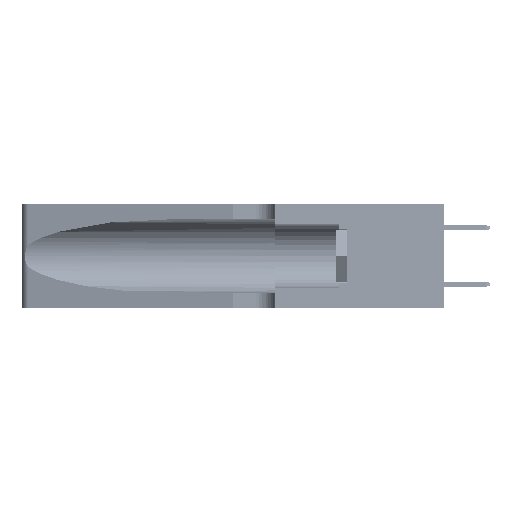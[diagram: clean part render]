
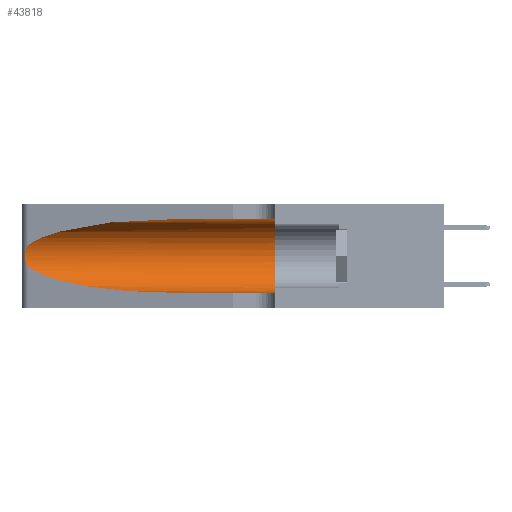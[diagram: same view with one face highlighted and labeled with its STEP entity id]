
A CAD part, left-side view. The second image highlights one B-rep face of the part: STEP entity #43818.
In plain terms, the highlighted cylindrical face has radius 3.308 mm (diameter 6.617 mm), a partial arc.
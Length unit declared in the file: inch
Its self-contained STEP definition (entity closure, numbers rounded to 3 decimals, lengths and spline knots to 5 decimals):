
#5 = AXIS2_PLACEMENT_3D ( 'NONE', #3185, #15823, #49027 ) ;
#410 = LINE ( 'NONE', #9595, #32547 ) ;
#458 = CARTESIAN_POINT ( 'NONE',  ( 0.2373, 1.15595, 0.08982 ) ) ;
#2467 = VERTEX_POINT ( 'NONE', #25370 ) ;
#3185 = CARTESIAN_POINT ( 'NONE',  ( 0.1305, 1.61858, 0.185 ) ) ;
#3196 = DIRECTION ( 'NONE',  ( 0., -1., 0. ) ) ;
#3624 = CARTESIAN_POINT ( 'NONE',  ( 0.25555, 1.22993, 0.14849 ) ) ;
#4055 = AXIS2_PLACEMENT_3D ( 'NONE', #11667, #40899, #15876 ) ;
#4737 = CARTESIAN_POINT ( 'NONE',  ( 0.18966, 0.96281, 0.05475 ) ) ;
#4950 = VERTEX_POINT ( 'NONE', #36254 ) ;
#5387 = B_SPLINE_CURVE_WITH_KNOTS ( 'NONE', 3,
 ( #49276, #53444, #36911, #11862, #41106, #16078, #45245, #20283, #49447, #24527, #53612, #28703, #3624, #32874 ),
 .UNSPECIFIED., .F., .F.,
 ( 4, 2, 2, 2, 2, 2, 4 ),
 ( 0., 0.00027, 0.00053, 0.00107, 0.0016, 0.00187, 0.00214 ),
 .UNSPECIFIED. ) ;
#6263 = CARTESIAN_POINT ( 'NONE',  ( 0.18966, 0.96281, 0.31525 ) ) ;
#9595 = CARTESIAN_POINT ( 'NONE',  ( 0.1305, 1.61858, 0.05475 ) ) ;
#11667 = CARTESIAN_POINT ( 'NONE',  ( 0.1305, 0.35, 0.185 ) ) ;
#11862 = CARTESIAN_POINT ( 'NONE',  ( 0.25787, 1.23484, 0.2124 ) ) ;
#15106 =( BOUNDED_CURVE ( )  B_SPLINE_CURVE ( 3, ( #39679, #6263, #43853, #18870 ),
 .UNSPECIFIED., .F., .F. ) 
 B_SPLINE_CURVE_WITH_KNOTS ( ( 4, 4 ),
 ( 1.5708, 2.84003 ),
 .UNSPECIFIED. ) 
 CURVE ( )  GEOMETRIC_REPRESENTATION_ITEM ( )  RATIONAL_B_SPLINE_CURVE ( ( 1., 0.87, 0.87, 1. ) ) 
 REPRESENTATION_ITEM ( '' )  );
#15823 = DIRECTION ( 'NONE',  ( 0., -1., 0. ) ) ;
#15876 = DIRECTION ( 'NONE',  ( 0., 0., 1. ) ) ;
#16078 = CARTESIAN_POINT ( 'NONE',  ( 0.26018, 1.23835, 0.19895 ) ) ;
#18870 = CARTESIAN_POINT ( 'NONE',  ( 0.25487, 1.22718, 0.22369 ) ) ;
#19521 = VERTEX_POINT ( 'NONE', #27948 ) ;
#20283 = CARTESIAN_POINT ( 'NONE',  ( 0.26075, 1.23896, 0.178 ) ) ;
#21993 = CARTESIAN_POINT ( 'NONE',  ( 0.1305, 0.35, 0.05475 ) ) ;
#24445 = ORIENTED_EDGE ( 'NONE', *, *, #25282, .F. ) ;
#24527 = CARTESIAN_POINT ( 'NONE',  ( 0.25856, 1.23593, 0.16098 ) ) ;
#25282 = EDGE_CURVE ( 'NONE', #19521, #28025, #32556, .T. ) ;
#25370 = CARTESIAN_POINT ( 'NONE',  ( 0.1305, 0.72297, 0.05475 ) ) ;
#26620 = CYLINDRICAL_SURFACE ( 'NONE', #5, 0.13025 ) ;
#26859 = ORIENTED_EDGE ( 'NONE', *, *, #36422, .T. ) ;
#27948 = CARTESIAN_POINT ( 'NONE',  ( 0.1305, 0.35, 0.31525 ) ) ;
#28025 = VERTEX_POINT ( 'NONE', #21993 ) ;
#28703 = CARTESIAN_POINT ( 'NONE',  ( 0.25639, 1.23186, 0.15144 ) ) ;
#29761 = CARTESIAN_POINT ( 'NONE',  ( 0.25487, 1.22718, 0.14631 ) ) ;
#30790 = ORIENTED_EDGE ( 'NONE', *, *, #38462, .T. ) ;
#32547 = VECTOR ( 'NONE', #39021, 39.37008 ) ;
#32556 = CIRCLE ( 'NONE', #4055, 0.13025 ) ;
#32762 = VERTEX_POINT ( 'NONE', #51958 ) ;
#32874 = CARTESIAN_POINT ( 'NONE',  ( 0.25487, 1.22718, 0.14631 ) ) ;
#33967 = CARTESIAN_POINT ( 'NONE',  ( 0.1305, 0.72297, 0.05475 ) ) ;
#33971 = EDGE_CURVE ( 'NONE', #4950, #32762, #15106, .T. ) ;
#35646 = EDGE_LOOP ( 'NONE', ( #36653, #26859, #30790, #45253, #24445, #37536 ) ) ;
#36254 = CARTESIAN_POINT ( 'NONE',  ( 0.1305, 0.72297, 0.31525 ) ) ;
#36422 = EDGE_CURVE ( 'NONE', #32762, #48910, #5387, .T. ) ;
#36653 = ORIENTED_EDGE ( 'NONE', *, *, #33971, .T. ) ;
#36667 = CARTESIAN_POINT ( 'NONE',  ( 0.1305, 1.61858, 0.31525 ) ) ;
#36911 = CARTESIAN_POINT ( 'NONE',  ( 0.25639, 1.23184, 0.21858 ) ) ;
#37184 = LINE ( 'NONE', #36667, #46931 ) ;
#37536 = ORIENTED_EDGE ( 'NONE', *, *, #48543, .F. ) ;
#38462 = EDGE_CURVE ( 'NONE', #48910, #2467, #49846, .T. ) ;
#39021 = DIRECTION ( 'NONE',  ( 0., -1., 0. ) ) ;
#39679 = CARTESIAN_POINT ( 'NONE',  ( 0.1305, 0.72297, 0.31525 ) ) ;
#40337 = FACE_OUTER_BOUND ( 'NONE', #35646, .T. ) ;
#40899 = DIRECTION ( 'NONE',  ( 0., 1., 0. ) ) ;
#41106 = CARTESIAN_POINT ( 'NONE',  ( 0.25854, 1.2359, 0.20912 ) ) ;
#43147 = CARTESIAN_POINT ( 'NONE',  ( 0.25487, 1.22718, 0.14631 ) ) ;
#43485 = EDGE_CURVE ( 'NONE', #2467, #28025, #410, .T. ) ;
#43818 = ADVANCED_FACE ( 'NONE', ( #40337 ), #26620, .F. ) ;
#43853 = CARTESIAN_POINT ( 'NONE',  ( 0.2373, 1.15595, 0.28018 ) ) ;
#45245 = CARTESIAN_POINT ( 'NONE',  ( 0.26075, 1.23896, 0.19203 ) ) ;
#45253 = ORIENTED_EDGE ( 'NONE', *, *, #43485, .T. ) ;
#46931 = VECTOR ( 'NONE', #3196, 39.37008 ) ;
#48543 = EDGE_CURVE ( 'NONE', #4950, #19521, #37184, .T. ) ;
#48910 = VERTEX_POINT ( 'NONE', #43147 ) ;
#49027 = DIRECTION ( 'NONE',  ( 0., 0., -1. ) ) ;
#49276 = CARTESIAN_POINT ( 'NONE',  ( 0.25487, 1.22718, 0.22369 ) ) ;
#49447 = CARTESIAN_POINT ( 'NONE',  ( 0.26017, 1.23833, 0.17102 ) ) ;
#49846 =( BOUNDED_CURVE ( )  B_SPLINE_CURVE ( 3, ( #29761, #458, #4737, #33967 ),
 .UNSPECIFIED., .F., .F. ) 
 B_SPLINE_CURVE_WITH_KNOTS ( ( 4, 4 ),
 ( 3.44316, 4.71239 ),
 .UNSPECIFIED. ) 
 CURVE ( )  GEOMETRIC_REPRESENTATION_ITEM ( )  RATIONAL_B_SPLINE_CURVE ( ( 1., 0.87, 0.87, 1. ) ) 
 REPRESENTATION_ITEM ( '' )  );
#51958 = CARTESIAN_POINT ( 'NONE',  ( 0.25487, 1.22718, 0.22369 ) ) ;
#53444 = CARTESIAN_POINT ( 'NONE',  ( 0.25555, 1.22994, 0.2215 ) ) ;
#53612 = CARTESIAN_POINT ( 'NONE',  ( 0.25789, 1.23486, 0.15765 ) ) ;
